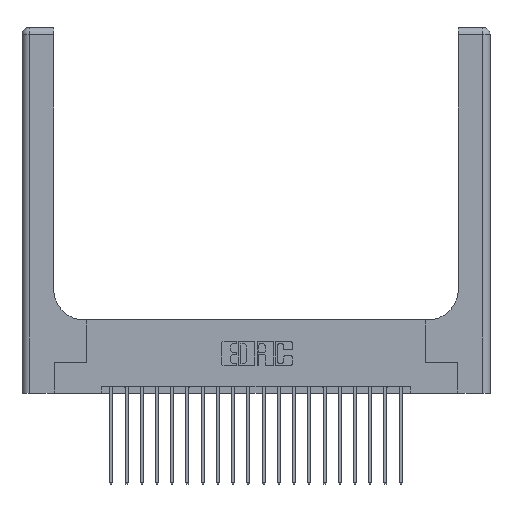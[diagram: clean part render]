
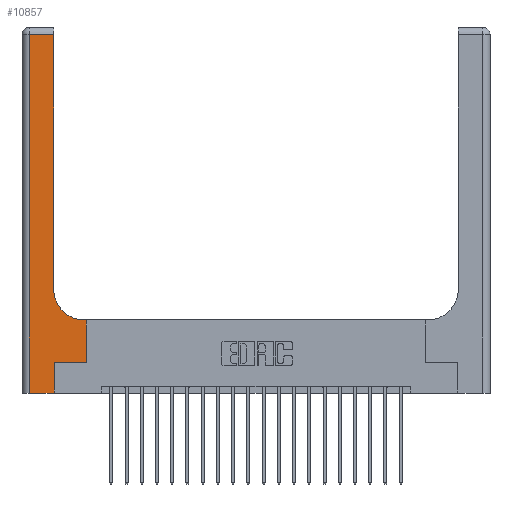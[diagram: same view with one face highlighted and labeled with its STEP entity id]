
A CAD part, top view. The second image highlights one B-rep face of the part: STEP entity #10857.
In plain terms, the highlighted planar face has unit normal (0, 0, 1).
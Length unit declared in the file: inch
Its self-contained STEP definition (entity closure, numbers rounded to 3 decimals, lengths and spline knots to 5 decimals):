
#94 = CARTESIAN_POINT ( 'NONE',  ( 0.265, 0., 0.37 ) ) ;
#126 = CARTESIAN_POINT ( 'NONE',  ( 0., 3., 0.37 ) ) ;
#135 = CARTESIAN_POINT ( 'NONE',  ( 0.265, 0., 0.37 ) ) ;
#142 = ORIENTED_EDGE ( 'NONE', *, *, #15958, .T. ) ;
#190 = LINE ( 'NONE', #15395, #12594 ) ;
#212 = CARTESIAN_POINT ( 'NONE',  ( 0.26, 0.85, 0.37 ) ) ;
#220 = CIRCLE ( 'NONE', #13879, 0.25 ) ;
#1097 = EDGE_LOOP ( 'NONE', ( #7621, #142, #15546, #15377, #5129, #7175, #2855, #3083, #7440 ) ) ;
#1686 = VERTEX_POINT ( 'NONE', #17457 ) ;
#1773 = VECTOR ( 'NONE', #10096, 39.37008 ) ;
#2714 = DIRECTION ( 'NONE',  ( 0., -1., 0. ) ) ;
#2855 = ORIENTED_EDGE ( 'NONE', *, *, #18165, .T. ) ;
#3083 = ORIENTED_EDGE ( 'NONE', *, *, #13512, .T. ) ;
#3437 = CARTESIAN_POINT ( 'NONE',  ( 0.528, 0.25, 0.37 ) ) ;
#3591 = VERTEX_POINT ( 'NONE', #17892 ) ;
#4142 = DIRECTION ( 'NONE',  ( 0., 0., -1. ) ) ;
#4174 = LINE ( 'NONE', #11253, #9606 ) ;
#4194 = CARTESIAN_POINT ( 'NONE',  ( 0.26, 2.94, 0.37 ) ) ;
#4335 = LINE ( 'NONE', #13474, #17687 ) ;
#4361 = LINE ( 'NONE', #11237, #11645 ) ;
#5129 = ORIENTED_EDGE ( 'NONE', *, *, #12825, .T. ) ;
#5325 = DIRECTION ( 'NONE',  ( 1., 0., 0. ) ) ;
#5964 = VERTEX_POINT ( 'NONE', #135 ) ;
#6161 = LINE ( 'NONE', #10020, #1773 ) ;
#6545 = VECTOR ( 'NONE', #19650, 39.37008 ) ;
#7045 = EDGE_CURVE ( 'NONE', #9441, #15527, #12005, .T. ) ;
#7175 = ORIENTED_EDGE ( 'NONE', *, *, #7045, .T. ) ;
#7267 = CARTESIAN_POINT ( 'NONE',  ( 0.51, 0.85, 0.37 ) ) ;
#7440 = ORIENTED_EDGE ( 'NONE', *, *, #18457, .T. ) ;
#7621 = ORIENTED_EDGE ( 'NONE', *, *, #10786, .T. ) ;
#7809 = DIRECTION ( 'NONE',  ( -1., 0., 0. ) ) ;
#7832 = VERTEX_POINT ( 'NONE', #8540 ) ;
#8120 = DIRECTION ( 'NONE',  ( 0., 0., -1. ) ) ;
#8540 = CARTESIAN_POINT ( 'NONE',  ( 0.51, 0.6, 0.37 ) ) ;
#8808 = EDGE_CURVE ( 'NONE', #1686, #19706, #4174, .T. ) ;
#9441 = VERTEX_POINT ( 'NONE', #14867 ) ;
#9606 = VECTOR ( 'NONE', #2714, 39.37008 ) ;
#9981 = DIRECTION ( 'NONE',  ( 0., 1., 0. ) ) ;
#10020 = CARTESIAN_POINT ( 'NONE',  ( 0.26, 3., 0.37 ) ) ;
#10021 = CARTESIAN_POINT ( 'NONE',  ( 0.528, 0.25, 0.37 ) ) ;
#10096 = DIRECTION ( 'NONE',  ( 0., 1., 0. ) ) ;
#10694 = DIRECTION ( 'NONE',  ( -1., 0., 0. ) ) ;
#10786 = EDGE_CURVE ( 'NONE', #20449, #17391, #6161, .T. ) ;
#10857 = ADVANCED_FACE ( 'NONE', ( #11083 ), #14746, .F. ) ;
#10913 = EDGE_CURVE ( 'NONE', #19706, #5964, #4335, .T. ) ;
#10961 = LINE ( 'NONE', #3437, #6545 ) ;
#11083 = FACE_OUTER_BOUND ( 'NONE', #1097, .T. ) ;
#11237 = CARTESIAN_POINT ( 'NONE',  ( 0.26, 0.6, 0.37 ) ) ;
#11253 = CARTESIAN_POINT ( 'NONE',  ( 0.06, 3., 0.37 ) ) ;
#11645 = VECTOR ( 'NONE', #7809, 39.37008 ) ;
#12005 = LINE ( 'NONE', #12294, #15801 ) ;
#12206 = DIRECTION ( 'NONE',  ( 1., 0., 0. ) ) ;
#12208 = LINE ( 'NONE', #94, #12435 ) ;
#12294 = CARTESIAN_POINT ( 'NONE',  ( 0.265, 0.25, 0.37 ) ) ;
#12435 = VECTOR ( 'NONE', #9981, 39.37008 ) ;
#12594 = VECTOR ( 'NONE', #10694, 39.37008 ) ;
#12825 = EDGE_CURVE ( 'NONE', #5964, #9441, #12208, .T. ) ;
#13474 = CARTESIAN_POINT ( 'NONE',  ( 0., 0., 0.37 ) ) ;
#13512 = EDGE_CURVE ( 'NONE', #3591, #7832, #4361, .T. ) ;
#13635 = DIRECTION ( 'NONE',  ( 1., 0., 0. ) ) ;
#13879 = AXIS2_PLACEMENT_3D ( 'NONE', #7267, #4142, #12206 ) ;
#14746 = PLANE ( 'NONE',  #18935 ) ;
#14816 = DIRECTION ( 'NONE',  ( -1., 0., 0. ) ) ;
#14867 = CARTESIAN_POINT ( 'NONE',  ( 0.265, 0.25, 0.37 ) ) ;
#15377 = ORIENTED_EDGE ( 'NONE', *, *, #10913, .T. ) ;
#15395 = CARTESIAN_POINT ( 'NONE',  ( 0., 2.94, 0.37 ) ) ;
#15527 = VERTEX_POINT ( 'NONE', #10021 ) ;
#15546 = ORIENTED_EDGE ( 'NONE', *, *, #8808, .T. ) ;
#15801 = VECTOR ( 'NONE', #13635, 39.37008 ) ;
#15931 = CARTESIAN_POINT ( 'NONE',  ( 0.06, 0., 0.37 ) ) ;
#15958 = EDGE_CURVE ( 'NONE', #17391, #1686, #190, .T. ) ;
#17391 = VERTEX_POINT ( 'NONE', #4194 ) ;
#17457 = CARTESIAN_POINT ( 'NONE',  ( 0.06, 2.94, 0.37 ) ) ;
#17687 = VECTOR ( 'NONE', #5325, 39.37008 ) ;
#17892 = CARTESIAN_POINT ( 'NONE',  ( 0.528, 0.6, 0.37 ) ) ;
#18165 = EDGE_CURVE ( 'NONE', #15527, #3591, #10961, .T. ) ;
#18457 = EDGE_CURVE ( 'NONE', #7832, #20449, #220, .T. ) ;
#18935 = AXIS2_PLACEMENT_3D ( 'NONE', #126, #8120, #14816 ) ;
#19650 = DIRECTION ( 'NONE',  ( 0., 1., 0. ) ) ;
#19706 = VERTEX_POINT ( 'NONE', #15931 ) ;
#20449 = VERTEX_POINT ( 'NONE', #212 ) ;
